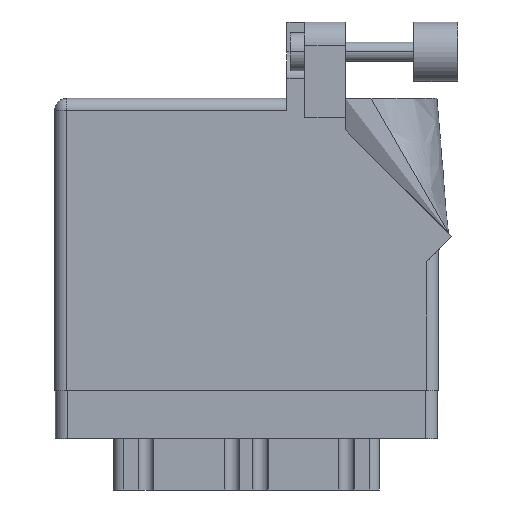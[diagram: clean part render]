
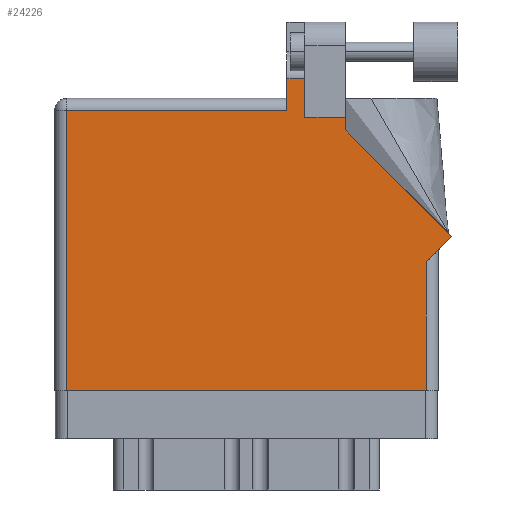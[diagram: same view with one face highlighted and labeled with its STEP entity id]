
A CAD part, front view. The second image highlights one B-rep face of the part: STEP entity #24226.
In plain terms, the highlighted face is planar.
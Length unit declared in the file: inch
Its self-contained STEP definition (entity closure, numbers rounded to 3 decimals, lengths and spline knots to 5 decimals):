
#378 = EDGE_CURVE ( 'NONE', #2850, #6122, #13925, .T. ) ;
#492 = CARTESIAN_POINT ( 'NONE',  ( 1.948, 0., 0. ) ) ;
#578 = CARTESIAN_POINT ( 'NONE',  ( 2.08071, 0.80771, 0. ) ) ;
#932 = ORIENTED_EDGE ( 'NONE', *, *, #4828, .T. ) ;
#1339 = DIRECTION ( 'NONE',  ( -0.707, 0.707, 0. ) ) ;
#1846 = EDGE_CURVE ( 'NONE', #33756, #20125, #7184, .T. ) ;
#1863 = CARTESIAN_POINT ( 'NONE',  ( 2.08071, 0.80771, 0. ) ) ;
#2574 = VERTEX_POINT ( 'NONE', #17997 ) ;
#2850 = VERTEX_POINT ( 'NONE', #22387 ) ;
#3178 = VECTOR ( 'NONE', #31227, 39.37008 ) ;
#4232 = ORIENTED_EDGE ( 'NONE', *, *, #378, .T. ) ;
#4758 = CARTESIAN_POINT ( 'NONE',  ( 1.64177, 1.6315, 0. ) ) ;
#4828 = EDGE_CURVE ( 'NONE', #2574, #33756, #7827, .T. ) ;
#5067 = ORIENTED_EDGE ( 'NONE', *, *, #1846, .T. ) ;
#5102 = CARTESIAN_POINT ( 'NONE',  ( 1.948, 0.737, 0. ) ) ;
#5175 = ORIENTED_EDGE ( 'NONE', *, *, #11348, .T. ) ;
#6122 = VERTEX_POINT ( 'NONE', #33716 ) ;
#6134 = DIRECTION ( 'NONE',  ( 0., -1., 0. ) ) ;
#6259 = ORIENTED_EDGE ( 'NONE', *, *, #18755, .T. ) ;
#6536 = ORIENTED_EDGE ( 'NONE', *, *, #6690, .T. ) ;
#6690 = EDGE_CURVE ( 'NONE', #27440, #8946, #13100, .T. ) ;
#7184 = LINE ( 'NONE', #1863, #15658 ) ;
#7220 = EDGE_CURVE ( 'NONE', #32051, #16873, #29843, .T. ) ;
#7353 = LINE ( 'NONE', #20445, #3178 ) ;
#7475 = DIRECTION ( 'NONE',  ( 0.707, 0.707, 0. ) ) ;
#7827 = LINE ( 'NONE', #18611, #22657 ) ;
#8617 = DIRECTION ( 'NONE',  ( 1., 0., 0. ) ) ;
#8693 = VERTEX_POINT ( 'NONE', #26475 ) ;
#8745 = VECTOR ( 'NONE', #6134, 39.37008 ) ;
#8946 = VERTEX_POINT ( 'NONE', #29632 ) ;
#9222 = CARTESIAN_POINT ( 'NONE',  ( 0., 1.53, 0. ) ) ;
#9597 = CARTESIAN_POINT ( 'NONE',  ( 1.524, 1.43, 0. ) ) ;
#9801 = LINE ( 'NONE', #12283, #34566 ) ;
#10118 = CARTESIAN_POINT ( 'NONE',  ( 0.062, 1.468, 0. ) ) ;
#10625 = DIRECTION ( 'NONE',  ( 0., 1., 0. ) ) ;
#10740 = EDGE_CURVE ( 'NONE', #20125, #8693, #19712, .T. ) ;
#11348 = EDGE_CURVE ( 'NONE', #8693, #27440, #29029, .T. ) ;
#11450 = CARTESIAN_POINT ( 'NONE',  ( 0., 0., 0. ) ) ;
#12283 = CARTESIAN_POINT ( 'NONE',  ( 0., 1.468, 0. ) ) ;
#12552 = EDGE_LOOP ( 'NONE', ( #6536, #24534, #4232, #6259, #13473, #30788, #26267, #932, #5067, #32730, #5175 ) ) ;
#13100 = LINE ( 'NONE', #23884, #30078 ) ;
#13473 = ORIENTED_EDGE ( 'NONE', *, *, #26841, .T. ) ;
#13925 = LINE ( 'NONE', #16937, #8745 ) ;
#14410 = CARTESIAN_POINT ( 'NONE',  ( 1.524, 1.36442, 0. ) ) ;
#15658 = VECTOR ( 'NONE', #1339, 39.37008 ) ;
#15678 = EDGE_CURVE ( 'NONE', #8946, #2850, #18199, .T. ) ;
#15903 = DIRECTION ( 'NONE',  ( 0., 1., 0. ) ) ;
#16873 = VERTEX_POINT ( 'NONE', #492 ) ;
#16937 = CARTESIAN_POINT ( 'NONE',  ( 1.217, 1.53, 0. ) ) ;
#17023 = DIRECTION ( 'NONE',  ( 0., 0., -1. ) ) ;
#17523 = VECTOR ( 'NONE', #28336, 39.37008 ) ;
#17997 = CARTESIAN_POINT ( 'NONE',  ( 1.948, 0.675, 0. ) ) ;
#18199 = LINE ( 'NONE', #4758, #25379 ) ;
#18611 = CARTESIAN_POINT ( 'NONE',  ( 2.01, 0.737, 0. ) ) ;
#18755 = EDGE_CURVE ( 'NONE', #6122, #25596, #9801, .T. ) ;
#19712 = LINE ( 'NONE', #14410, #28736 ) ;
#20125 = VERTEX_POINT ( 'NONE', #29596 ) ;
#20445 = CARTESIAN_POINT ( 'NONE',  ( 0.062, 0., 0. ) ) ;
#20578 = DIRECTION ( 'NONE',  ( -1., 0., 0. ) ) ;
#22387 = CARTESIAN_POINT ( 'NONE',  ( 1.217, 1.6315, 0. ) ) ;
#22657 = VECTOR ( 'NONE', #7475, 39.37008 ) ;
#23884 = CARTESIAN_POINT ( 'NONE',  ( 1.311, 1.43, 0. ) ) ;
#24113 = CARTESIAN_POINT ( 'NONE',  ( 1.311, 1.43, 0. ) ) ;
#24226 = ADVANCED_FACE ( 'NONE', ( #25148 ), #25855, .F. ) ;
#24534 = ORIENTED_EDGE ( 'NONE', *, *, #15678, .T. ) ;
#24948 = EDGE_CURVE ( 'NONE', #16873, #2574, #32149, .T. ) ;
#25148 = FACE_OUTER_BOUND ( 'NONE', #12552, .T. ) ;
#25378 = DIRECTION ( 'NONE',  ( 0., 1., 0. ) ) ;
#25377 = CARTESIAN_POINT ( 'NONE',  ( 0.062, 0., 0. ) ) ;
#25379 = VECTOR ( 'NONE', #26351, 39.37008 ) ;
#25596 = VERTEX_POINT ( 'NONE', #10118 ) ;
#25855 = PLANE ( 'NONE',  #26359 ) ;
#26267 = ORIENTED_EDGE ( 'NONE', *, *, #24948, .T. ) ;
#26351 = DIRECTION ( 'NONE',  ( -1., 0., 0. ) ) ;
#26359 = AXIS2_PLACEMENT_3D ( 'NONE', #9222, #17023, #30624 ) ;
#26475 = CARTESIAN_POINT ( 'NONE',  ( 1.524, 1.43, 0. ) ) ;
#26841 = EDGE_CURVE ( 'NONE', #25596, #32051, #7353, .T. ) ;
#27440 = VERTEX_POINT ( 'NONE', #24113 ) ;
#28336 = DIRECTION ( 'NONE',  ( -1., 0., 0. ) ) ;
#28635 = VECTOR ( 'NONE', #15903, 39.37008 ) ;
#28736 = VECTOR ( 'NONE', #25378, 39.37008 ) ;
#29029 = LINE ( 'NONE', #9597, #17523 ) ;
#29596 = CARTESIAN_POINT ( 'NONE',  ( 1.524, 1.36442, 0. ) ) ;
#29632 = CARTESIAN_POINT ( 'NONE',  ( 1.311, 1.6315, 0. ) ) ;
#29843 = LINE ( 'NONE', #11450, #33535 ) ;
#30078 = VECTOR ( 'NONE', #10625, 39.37008 ) ;
#30624 = DIRECTION ( 'NONE',  ( -1., 0., 0. ) ) ;
#30788 = ORIENTED_EDGE ( 'NONE', *, *, #7220, .T. ) ;
#31227 = DIRECTION ( 'NONE',  ( 0., -1., 0. ) ) ;
#32051 = VERTEX_POINT ( 'NONE', #25377 ) ;
#32149 = LINE ( 'NONE', #5102, #28635 ) ;
#32730 = ORIENTED_EDGE ( 'NONE', *, *, #10740, .T. ) ;
#33535 = VECTOR ( 'NONE', #8617, 39.37008 ) ;
#33716 = CARTESIAN_POINT ( 'NONE',  ( 1.217, 1.468, 0. ) ) ;
#33756 = VERTEX_POINT ( 'NONE', #578 ) ;
#34566 = VECTOR ( 'NONE', #20578, 39.37008 ) ;
